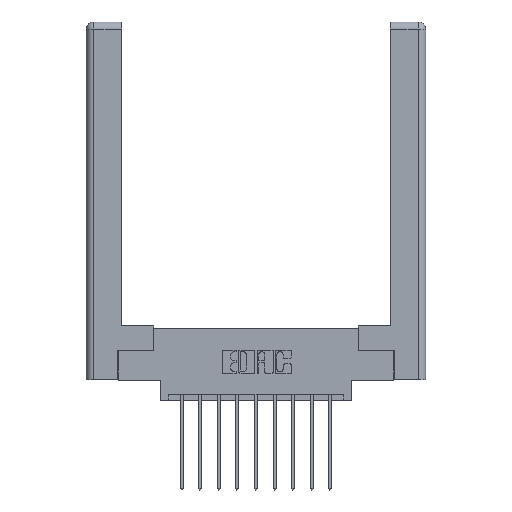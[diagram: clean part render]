
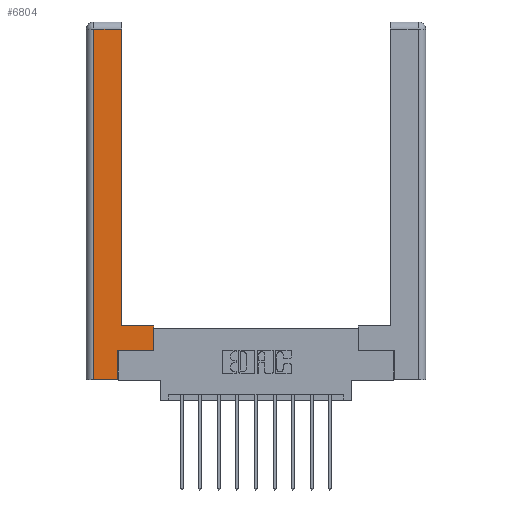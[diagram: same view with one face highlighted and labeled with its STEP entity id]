
A CAD part, top view. The second image highlights one B-rep face of the part: STEP entity #6804.
In plain terms, the highlighted planar face has unit normal (0, 0, 1).
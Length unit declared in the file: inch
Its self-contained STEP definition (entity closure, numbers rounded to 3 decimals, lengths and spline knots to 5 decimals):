
#79 = ORIENTED_EDGE ( 'NONE', *, *, #8279, .T. ) ;
#88 = DIRECTION ( 'NONE',  ( -1., 0., 0. ) ) ;
#810 = LINE ( 'NONE', #5566, #11505 ) ;
#1097 = EDGE_CURVE ( 'NONE', #11981, #4740, #1996, .T. ) ;
#1558 = CARTESIAN_POINT ( 'NONE',  ( 0.565, 0.245, 0. ) ) ;
#1586 = VERTEX_POINT ( 'NONE', #6832 ) ;
#1860 = CARTESIAN_POINT ( 'NONE',  ( 0.265, 0., 0. ) ) ;
#1939 = LINE ( 'NONE', #12626, #5862 ) ;
#1955 = CARTESIAN_POINT ( 'NONE',  ( 0.0615, 0., 0. ) ) ;
#1996 = LINE ( 'NONE', #4841, #13873 ) ;
#2045 = DIRECTION ( 'NONE',  ( 0., 0., -1. ) ) ;
#2297 = EDGE_CURVE ( 'NONE', #10657, #3073, #810, .T. ) ;
#2663 = ORIENTED_EDGE ( 'NONE', *, *, #2297, .T. ) ;
#2711 = ORIENTED_EDGE ( 'NONE', *, *, #13870, .T. ) ;
#2721 = CARTESIAN_POINT ( 'NONE',  ( 0.0615, 0., 0. ) ) ;
#3073 = VERTEX_POINT ( 'NONE', #12756 ) ;
#3274 = CARTESIAN_POINT ( 'NONE',  ( 0.265, 0., 0. ) ) ;
#3516 = VECTOR ( 'NONE', #9251, 39.37008 ) ;
#3536 = VECTOR ( 'NONE', #4090, 39.37008 ) ;
#4090 = DIRECTION ( 'NONE',  ( 0., -1., 0. ) ) ;
#4173 = DIRECTION ( 'NONE',  ( -1., 0., 0. ) ) ;
#4366 = LINE ( 'NONE', #1558, #6890 ) ;
#4508 = EDGE_CURVE ( 'NONE', #4740, #5452, #1939, .T. ) ;
#4740 = VERTEX_POINT ( 'NONE', #8264 ) ;
#4841 = CARTESIAN_POINT ( 'NONE',  ( 0.565, 0.45, 0. ) ) ;
#5224 = ORIENTED_EDGE ( 'NONE', *, *, #8269, .T. ) ;
#5452 = VERTEX_POINT ( 'NONE', #11307 ) ;
#5566 = CARTESIAN_POINT ( 'NONE',  ( 0.0615, 2.94, 0. ) ) ;
#5862 = VECTOR ( 'NONE', #10945, 39.37008 ) ;
#6624 = AXIS2_PLACEMENT_3D ( 'NONE', #7440, #2045, #4173 ) ;
#6804 = ADVANCED_FACE ( 'NONE', ( #11603 ), #9667, .F. ) ;
#6832 = CARTESIAN_POINT ( 'NONE',  ( 0.265, 0.245, 0. ) ) ;
#6890 = VECTOR ( 'NONE', #11874, 39.37008 ) ;
#6975 = CARTESIAN_POINT ( 'NONE',  ( 0.295, 3., 0. ) ) ;
#7153 = ORIENTED_EDGE ( 'NONE', *, *, #4508, .T. ) ;
#7440 = CARTESIAN_POINT ( 'NONE',  ( 0., 0., 0. ) ) ;
#7480 = VECTOR ( 'NONE', #13144, 39.37008 ) ;
#7549 = EDGE_CURVE ( 'NONE', #11124, #1586, #7983, .T. ) ;
#7879 = EDGE_LOOP ( 'NONE', ( #5224, #2663, #2711, #11500, #12374, #79, #8329, #7153 ) ) ;
#7983 = LINE ( 'NONE', #13095, #7480 ) ;
#8259 = DIRECTION ( 'NONE',  ( 1., 0., 0. ) ) ;
#8264 = CARTESIAN_POINT ( 'NONE',  ( 0.565, 0.45, 0. ) ) ;
#8269 = EDGE_CURVE ( 'NONE', #5452, #10657, #9436, .T. ) ;
#8279 = EDGE_CURVE ( 'NONE', #1586, #11981, #4366, .T. ) ;
#8329 = ORIENTED_EDGE ( 'NONE', *, *, #1097, .T. ) ;
#8427 = LINE ( 'NONE', #1955, #3536 ) ;
#9061 = VECTOR ( 'NONE', #8259, 39.37008 ) ;
#9251 = DIRECTION ( 'NONE',  ( 0., 1., 0. ) ) ;
#9436 = LINE ( 'NONE', #6975, #3516 ) ;
#9476 = EDGE_CURVE ( 'NONE', #10574, #11124, #11969, .T. ) ;
#9667 = PLANE ( 'NONE',  #6624 ) ;
#10457 = CARTESIAN_POINT ( 'NONE',  ( 0.565, 0.245, 0. ) ) ;
#10574 = VERTEX_POINT ( 'NONE', #2721 ) ;
#10657 = VERTEX_POINT ( 'NONE', #12352 ) ;
#10945 = DIRECTION ( 'NONE',  ( -1., 0., 0. ) ) ;
#11124 = VERTEX_POINT ( 'NONE', #3274 ) ;
#11307 = CARTESIAN_POINT ( 'NONE',  ( 0.295, 0.45, 0. ) ) ;
#11500 = ORIENTED_EDGE ( 'NONE', *, *, #9476, .T. ) ;
#11505 = VECTOR ( 'NONE', #88, 39.37008 ) ;
#11603 = FACE_OUTER_BOUND ( 'NONE', #7879, .T. ) ;
#11874 = DIRECTION ( 'NONE',  ( 1., 0., 0. ) ) ;
#11969 = LINE ( 'NONE', #1860, #9061 ) ;
#11981 = VERTEX_POINT ( 'NONE', #10457 ) ;
#12352 = CARTESIAN_POINT ( 'NONE',  ( 0.295, 2.94, 0. ) ) ;
#12374 = ORIENTED_EDGE ( 'NONE', *, *, #7549, .T. ) ;
#12394 = DIRECTION ( 'NONE',  ( 0., 1., 0. ) ) ;
#12626 = CARTESIAN_POINT ( 'NONE',  ( 0.295, 0.45, 0. ) ) ;
#12756 = CARTESIAN_POINT ( 'NONE',  ( 0.0615, 2.94, 0. ) ) ;
#13095 = CARTESIAN_POINT ( 'NONE',  ( 0.265, 0.245, 0. ) ) ;
#13144 = DIRECTION ( 'NONE',  ( 0., 1., 0. ) ) ;
#13870 = EDGE_CURVE ( 'NONE', #3073, #10574, #8427, .T. ) ;
#13873 = VECTOR ( 'NONE', #12394, 39.37008 ) ;
